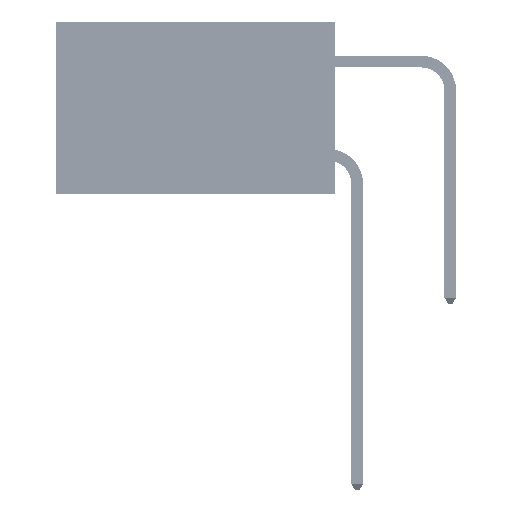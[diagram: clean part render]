
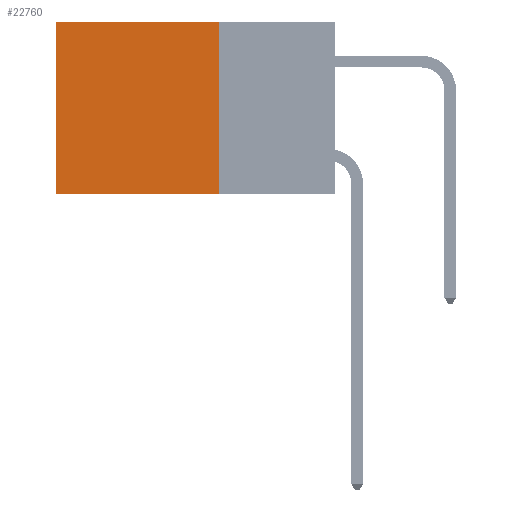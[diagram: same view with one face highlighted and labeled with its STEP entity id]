
A CAD part, left-side view. The second image highlights one B-rep face of the part: STEP entity #22760.
In plain terms, the highlighted planar face has unit normal (-1, 0, 0).
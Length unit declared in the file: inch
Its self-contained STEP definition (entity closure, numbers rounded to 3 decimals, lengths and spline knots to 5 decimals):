
#384 = CARTESIAN_POINT ( 'NONE',  ( 0.2875, 0.25, -0.37 ) ) ;
#2011 = VECTOR ( 'NONE', #2027, 39.37008 ) ;
#2027 = DIRECTION ( 'NONE',  ( 0., 0., -1. ) ) ;
#7224 = EDGE_CURVE ( 'NONE', #41521, #22451, #42345, .T. ) ;
#7225 = DIRECTION ( 'NONE',  ( 0., 0., -1. ) ) ;
#10062 = DIRECTION ( 'NONE',  ( 0., 0., -1. ) ) ;
#10300 = FACE_OUTER_BOUND ( 'NONE', #29852, .T. ) ;
#10999 = DIRECTION ( 'NONE',  ( 1., 0., 0. ) ) ;
#11409 = VERTEX_POINT ( 'NONE', #384 ) ;
#11774 = ORIENTED_EDGE ( 'NONE', *, *, #31428, .T. ) ;
#13161 = LINE ( 'NONE', #34457, #2011 ) ;
#13692 = DIRECTION ( 'NONE',  ( 0., 1., 0. ) ) ;
#16693 = CARTESIAN_POINT ( 'NONE',  ( 0.2875, 0.6, 0. ) ) ;
#16940 = ORIENTED_EDGE ( 'NONE', *, *, #7224, .T. ) ;
#19904 = ORIENTED_EDGE ( 'NONE', *, *, #21227, .F. ) ;
#20422 = VECTOR ( 'NONE', #36283, 39.37008 ) ;
#20712 = LINE ( 'NONE', #16693, #22625 ) ;
#21227 = EDGE_CURVE ( 'NONE', #41521, #11409, #13161, .T. ) ;
#21373 = LINE ( 'NONE', #32493, #20422 ) ;
#21520 = VECTOR ( 'NONE', #13692, 39.37008 ) ;
#22451 = VERTEX_POINT ( 'NONE', #37110 ) ;
#22625 = VECTOR ( 'NONE', #10062, 39.37008 ) ;
#22760 = ADVANCED_FACE ( 'NONE', ( #10300 ), #43428, .F. ) ;
#29329 = AXIS2_PLACEMENT_3D ( 'NONE', #46745, #10999, #7225 ) ;
#29852 = EDGE_LOOP ( 'NONE', ( #11774, #36225, #19904, #16940 ) ) ;
#31428 = EDGE_CURVE ( 'NONE', #22451, #34930, #20712, .T. ) ;
#32493 = CARTESIAN_POINT ( 'NONE',  ( 0.2875, 0.25, -0.37 ) ) ;
#33926 = EDGE_CURVE ( 'NONE', #11409, #34930, #21373, .T. ) ;
#34457 = CARTESIAN_POINT ( 'NONE',  ( 0.2875, 0.25, 0. ) ) ;
#34930 = VERTEX_POINT ( 'NONE', #36116 ) ;
#36116 = CARTESIAN_POINT ( 'NONE',  ( 0.2875, 0.6, -0.37 ) ) ;
#36225 = ORIENTED_EDGE ( 'NONE', *, *, #33926, .F. ) ;
#36283 = DIRECTION ( 'NONE',  ( 0., 1., 0. ) ) ;
#37110 = CARTESIAN_POINT ( 'NONE',  ( 0.2875, 0.6, 0. ) ) ;
#41377 = CARTESIAN_POINT ( 'NONE',  ( 0.2875, 0.25, 0. ) ) ;
#41521 = VERTEX_POINT ( 'NONE', #41377 ) ;
#42110 = CARTESIAN_POINT ( 'NONE',  ( 0.2875, 0.25, 0. ) ) ;
#42345 = LINE ( 'NONE', #42110, #21520 ) ;
#43428 = PLANE ( 'NONE',  #29329 ) ;
#46745 = CARTESIAN_POINT ( 'NONE',  ( 0.2875, 0.25, 0. ) ) ;
